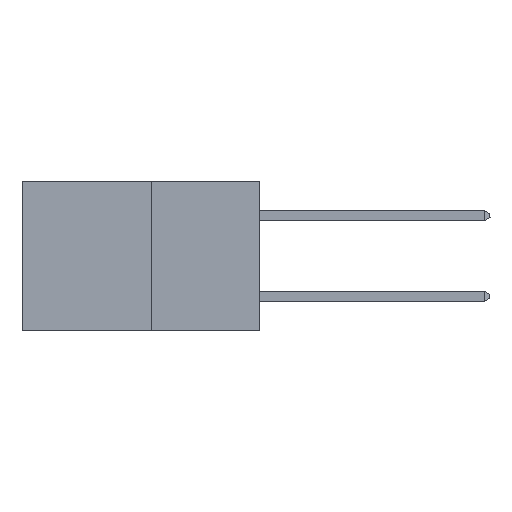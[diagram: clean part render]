
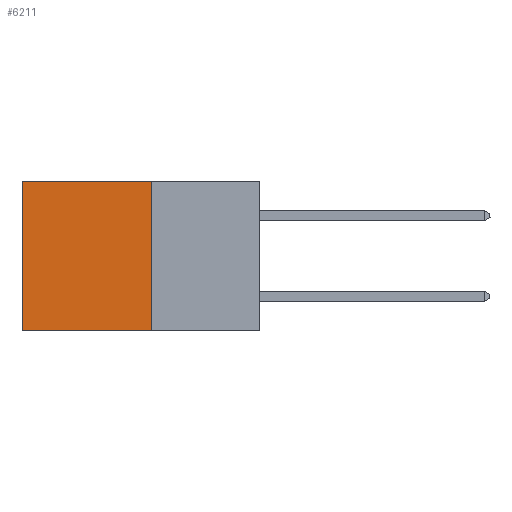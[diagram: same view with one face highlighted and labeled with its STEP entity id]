
A CAD part, left-side view. The second image highlights one B-rep face of the part: STEP entity #6211.
In plain terms, the highlighted planar face has unit normal (-1, 0, 0).
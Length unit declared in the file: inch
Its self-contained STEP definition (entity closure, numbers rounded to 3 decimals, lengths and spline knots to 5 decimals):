
#331 = EDGE_CURVE ( 'NONE', #19332, #20062, #18429, .T. ) ;
#744 = VECTOR ( 'NONE', #9541, 39.37008 ) ;
#849 = VERTEX_POINT ( 'NONE', #16460 ) ;
#3047 = DIRECTION ( 'NONE',  ( 0., 1., 0. ) ) ;
#3330 = VERTEX_POINT ( 'NONE', #28046 ) ;
#3684 = ORIENTED_EDGE ( 'NONE', *, *, #331, .T. ) ;
#3868 = EDGE_LOOP ( 'NONE', ( #23012, #17929, #19789, #3684 ) ) ;
#4441 = PLANE ( 'NONE',  #21998 ) ;
#5589 = CARTESIAN_POINT ( 'NONE',  ( 0.277, 0.27, 0. ) ) ;
#6211 = ADVANCED_FACE ( 'NONE', ( #25021 ), #4441, .F. ) ;
#6697 = VECTOR ( 'NONE', #3047, 39.37008 ) ;
#6935 = CARTESIAN_POINT ( 'NONE',  ( 0.277, 0.27, -0.37 ) ) ;
#7481 = LINE ( 'NONE', #27307, #6697 ) ;
#9123 = EDGE_CURVE ( 'NONE', #20062, #849, #20315, .T. ) ;
#9393 = DIRECTION ( 'NONE',  ( 0., 0., -1. ) ) ;
#9541 = DIRECTION ( 'NONE',  ( 0., 0., -1. ) ) ;
#9808 = CARTESIAN_POINT ( 'NONE',  ( 0.277, 0.27, -0.37 ) ) ;
#13294 = EDGE_CURVE ( 'NONE', #3330, #849, #7481, .T. ) ;
#13400 = CARTESIAN_POINT ( 'NONE',  ( 0.277, 0.59, 0. ) ) ;
#13765 = EDGE_CURVE ( 'NONE', #19332, #3330, #23786, .T. ) ;
#16460 = CARTESIAN_POINT ( 'NONE',  ( 0.277, 0.59, -0.37 ) ) ;
#17929 = ORIENTED_EDGE ( 'NONE', *, *, #13294, .F. ) ;
#18429 = LINE ( 'NONE', #20808, #24848 ) ;
#19143 = DIRECTION ( 'NONE',  ( 0., 1., 0. ) ) ;
#19332 = VERTEX_POINT ( 'NONE', #5589 ) ;
#19789 = ORIENTED_EDGE ( 'NONE', *, *, #13765, .F. ) ;
#20062 = VERTEX_POINT ( 'NONE', #13400 ) ;
#20315 = LINE ( 'NONE', #21752, #744 ) ;
#20808 = CARTESIAN_POINT ( 'NONE',  ( 0.277, 0.27, 0. ) ) ;
#21752 = CARTESIAN_POINT ( 'NONE',  ( 0.277, 0.59, -0.37 ) ) ;
#21919 = DIRECTION ( 'NONE',  ( 0., 0., -1. ) ) ;
#21998 = AXIS2_PLACEMENT_3D ( 'NONE', #6935, #23941, #9393 ) ;
#23012 = ORIENTED_EDGE ( 'NONE', *, *, #9123, .T. ) ;
#23786 = LINE ( 'NONE', #9808, #30197 ) ;
#23941 = DIRECTION ( 'NONE',  ( 1., 0., 0. ) ) ;
#24848 = VECTOR ( 'NONE', #19143, 39.37008 ) ;
#25021 = FACE_OUTER_BOUND ( 'NONE', #3868, .T. ) ;
#27307 = CARTESIAN_POINT ( 'NONE',  ( 0.277, 0.27, -0.37 ) ) ;
#28046 = CARTESIAN_POINT ( 'NONE',  ( 0.277, 0.27, -0.37 ) ) ;
#30197 = VECTOR ( 'NONE', #21919, 39.37008 ) ;
